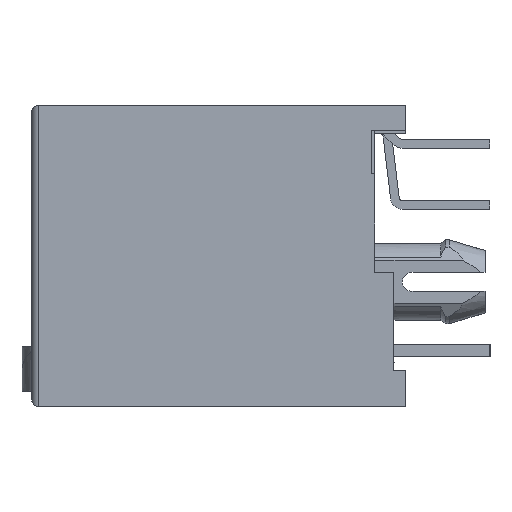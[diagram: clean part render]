
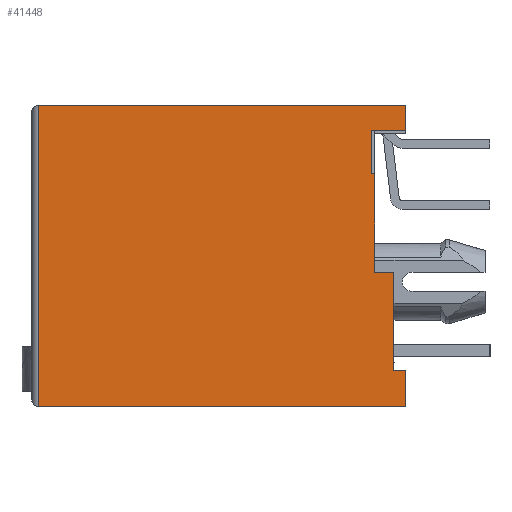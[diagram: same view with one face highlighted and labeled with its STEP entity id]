
A CAD part, left-side view. The second image highlights one B-rep face of the part: STEP entity #41448.
In plain terms, the highlighted planar face has unit normal (-1, 0, 0).
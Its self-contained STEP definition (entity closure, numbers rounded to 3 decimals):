
#1289 = CARTESIAN_POINT ( 'NONE',  ( -31.5, -7.8, -4.75 ) ) ;
#1361 = CARTESIAN_POINT ( 'NONE',  ( -31.5, -7.3, -2.017 ) ) ;
#2242 = ORIENTED_EDGE ( 'NONE', *, *, #23222, .F. ) ;
#2690 = CARTESIAN_POINT ( 'NONE',  ( -31.5, -7.8, 5.25 ) ) ;
#2831 = VERTEX_POINT ( 'NONE', #45628 ) ;
#3035 = VERTEX_POINT ( 'NONE', #38251 ) ;
#3059 = CARTESIAN_POINT ( 'NONE',  ( -31.5, -7.8, -4.75 ) ) ;
#3420 = CARTESIAN_POINT ( 'NONE',  ( -31.5, 2.4, -6.25 ) ) ;
#4001 = CARTESIAN_POINT ( 'NONE',  ( -31.5, -6.35, 3.45 ) ) ;
#9005 = VERTEX_POINT ( 'NONE', #67894 ) ;
#9206 = CARTESIAN_POINT ( 'NONE',  ( -31.5, -7.033, -0.65 ) ) ;
#9607 = EDGE_CURVE ( 'NONE', #9005, #52821, #56944, .T. ) ;
#10923 = B_SPLINE_CURVE_WITH_KNOTS ( 'NONE', 3,
 ( #65220, #17979, #29176, #18321 ),
 .UNSPECIFIED., .F., .F.,
 ( 4, 4 ),
 ( 0., 1. ),
 .UNSPECIFIED. ) ;
#11997 = ORIENTED_EDGE ( 'NONE', *, *, #55555, .F. ) ;
#12264 = ORIENTED_EDGE ( 'NONE', *, *, #9607, .F. ) ;
#12974 = EDGE_CURVE ( 'NONE', #28964, #3035, #21180, .T. ) ;
#13298 = ORIENTED_EDGE ( 'NONE', *, *, #45042, .F. ) ;
#13958 = CARTESIAN_POINT ( 'NONE',  ( -31.5, -7.8, -6.25 ) ) ;
#14138 = DIRECTION ( 'NONE',  ( 1., 0., 0. ) ) ;
#15414 = VERTEX_POINT ( 'NONE', #3059 ) ;
#15849 = EDGE_LOOP ( 'NONE', ( #11997, #13298, #56717, #12264, #29305, #52964, #27639, #54997, #2242, #47644, #48200, #30261 ) ) ;
#16614 = CARTESIAN_POINT ( 'NONE',  ( -31.5, -6.5, 3.45 ) ) ;
#16707 = B_SPLINE_CURVE_WITH_KNOTS ( 'NONE', 3,
 ( #13958, #35323, #3420, #68172 ),
 .UNSPECIFIED., .F., .F.,
 ( 4, 4 ),
 ( 0., 1. ),
 .UNSPECIFIED. ) ;
#17415 = CARTESIAN_POINT ( 'NONE',  ( -31.5, -7.633, -4.75 ) ) ;
#17540 = VERTEX_POINT ( 'NONE', #36992 ) ;
#17979 = CARTESIAN_POINT ( 'NONE',  ( -31.5, 7.5, 2.117 ) ) ;
#18321 = CARTESIAN_POINT ( 'NONE',  ( -31.5, 7.5, -6.25 ) ) ;
#18712 = FACE_OUTER_BOUND ( 'NONE', #15849, .T. ) ;
#19051 = EDGE_CURVE ( 'NONE', #2831, #23080, #10923, .T. ) ;
#19478 = EDGE_CURVE ( 'NONE', #65992, #2831, #42537, .T. ) ;
#19932 = CARTESIAN_POINT ( 'NONE',  ( -31.5, -6.45, 3.45 ) ) ;
#20110 = CARTESIAN_POINT ( 'NONE',  ( -31.5, -6.35, 5.25 ) ) ;
#20282 = CARTESIAN_POINT ( 'NONE',  ( -31.5, -6.4, 3.45 ) ) ;
#21180 = B_SPLINE_CURVE_WITH_KNOTS ( 'NONE', 3,
 ( #2690, #21926, #26493, #47478 ),
 .UNSPECIFIED., .F., .F.,
 ( 4, 4 ),
 ( 0., 1. ),
 .UNSPECIFIED. ) ;
#21926 = CARTESIAN_POINT ( 'NONE',  ( -31.5, -7.317, 5.25 ) ) ;
#22568 = CARTESIAN_POINT ( 'NONE',  ( -31.5, -7.8, 5.95 ) ) ;
#23080 = VERTEX_POINT ( 'NONE', #69085 ) ;
#23222 = EDGE_CURVE ( 'NONE', #65992, #28964, #29611, .T. ) ;
#23573 = EDGE_CURVE ( 'NONE', #52821, #56910, #57981, .T. ) ;
#23667 = CARTESIAN_POINT ( 'NONE',  ( -31.5, -7.8, -5.75 ) ) ;
#23926 = CARTESIAN_POINT ( 'NONE',  ( -31.5, -7.8, 5.25 ) ) ;
#25589 = CARTESIAN_POINT ( 'NONE',  ( -31.5, -6.35, 3.45 ) ) ;
#26236 = B_SPLINE_CURVE_WITH_KNOTS ( 'NONE', 3,
 ( #20110, #56537, #62806, #4001 ),
 .UNSPECIFIED., .F., .F.,
 ( 4, 4 ),
 ( 0., 1. ),
 .UNSPECIFIED. ) ;
#26493 = CARTESIAN_POINT ( 'NONE',  ( -31.5, -6.833, 5.25 ) ) ;
#26725 = EDGE_CURVE ( 'NONE', #44472, #47911, #36726, .T. ) ;
#27639 = ORIENTED_EDGE ( 'NONE', *, *, #55695, .F. ) ;
#28177 = CARTESIAN_POINT ( 'NONE',  ( -31.5, -7.8, 5.25 ) ) ;
#28919 = CARTESIAN_POINT ( 'NONE',  ( -31.5, -7.8, -5.25 ) ) ;
#28964 = VERTEX_POINT ( 'NONE', #23926 ) ;
#29176 = CARTESIAN_POINT ( 'NONE',  ( -31.5, 7.5, -2.067 ) ) ;
#29305 = ORIENTED_EDGE ( 'NONE', *, *, #69170, .F. ) ;
#29611 = B_SPLINE_CURVE_WITH_KNOTS ( 'NONE', 3,
 ( #58958, #22568, #43231, #28177 ),
 .UNSPECIFIED., .F., .F.,
 ( 4, 4 ),
 ( 0., 1. ),
 .UNSPECIFIED. ) ;
#30261 = ORIENTED_EDGE ( 'NONE', *, *, #34553, .F. ) ;
#31166 = AXIS2_PLACEMENT_3D ( 'NONE', #40754, #14138, #35502 ) ;
#33802 = CARTESIAN_POINT ( 'NONE',  ( -31.5, -6.5, 0.717 ) ) ;
#34553 = EDGE_CURVE ( 'NONE', #17540, #23080, #16707, .T. ) ;
#35323 = CARTESIAN_POINT ( 'NONE',  ( -31.5, -2.7, -6.25 ) ) ;
#35502 = DIRECTION ( 'NONE',  ( 0., 0., 1. ) ) ;
#35832 = CARTESIAN_POINT ( 'NONE',  ( -31.5, -6.5, -0.65 ) ) ;
#36726 = B_SPLINE_CURVE_WITH_KNOTS ( 'NONE', 3,
 ( #68205, #20282, #19932, #68551 ),
 .UNSPECIFIED., .F., .F.,
 ( 4, 4 ),
 ( 0., 1. ),
 .UNSPECIFIED. ) ;
#36861 = CARTESIAN_POINT ( 'NONE',  ( -31.5, -7.3, -0.65 ) ) ;
#36992 = CARTESIAN_POINT ( 'NONE',  ( -31.5, -7.8, -6.25 ) ) ;
#38251 = CARTESIAN_POINT ( 'NONE',  ( -31.5, -6.35, 5.25 ) ) ;
#38496 = CARTESIAN_POINT ( 'NONE',  ( -31.5, -7.3, -4.75 ) ) ;
#38780 = CARTESIAN_POINT ( 'NONE',  ( -31.5, -7.467, -4.75 ) ) ;
#39735 = CARTESIAN_POINT ( 'NONE',  ( -31.5, -6.5, -0.65 ) ) ;
#40754 = CARTESIAN_POINT ( 'NONE',  ( -31.5, 7.806, -6.501 ) ) ;
#41448 = ADVANCED_FACE ( 'NONE', ( #18712 ), #61732, .F. ) ;
#42120 = CARTESIAN_POINT ( 'NONE',  ( -31.5, 7.5, 6.3 ) ) ;
#42537 = B_SPLINE_CURVE_WITH_KNOTS ( 'NONE', 3,
 ( #46295, #63077, #62734, #42120 ),
 .UNSPECIFIED., .F., .F.,
 ( 4, 4 ),
 ( 0., 1. ),
 .UNSPECIFIED. ) ;
#43231 = CARTESIAN_POINT ( 'NONE',  ( -31.5, -7.8, 5.6 ) ) ;
#44472 = VERTEX_POINT ( 'NONE', #25589 ) ;
#45042 = EDGE_CURVE ( 'NONE', #56910, #15414, #51610, .T. ) ;
#45628 = CARTESIAN_POINT ( 'NONE',  ( -31.5, 7.5, 6.3 ) ) ;
#45699 = CARTESIAN_POINT ( 'NONE',  ( -31.5, -7.8, -4.75 ) ) ;
#46295 = CARTESIAN_POINT ( 'NONE',  ( -31.5, -7.8, 6.3 ) ) ;
#47478 = CARTESIAN_POINT ( 'NONE',  ( -31.5, -6.35, 5.25 ) ) ;
#47644 = ORIENTED_EDGE ( 'NONE', *, *, #19478, .T. ) ;
#47911 = VERTEX_POINT ( 'NONE', #16614 ) ;
#48200 = ORIENTED_EDGE ( 'NONE', *, *, #19051, .T. ) ;
#49001 = CARTESIAN_POINT ( 'NONE',  ( -31.5, -7.3, -0.65 ) ) ;
#49268 = CARTESIAN_POINT ( 'NONE',  ( -31.5, -7.3, -4.75 ) ) ;
#50349 = CARTESIAN_POINT ( 'NONE',  ( -31.5, -7.3, -3.383 ) ) ;
#50574 = CARTESIAN_POINT ( 'NONE',  ( -31.5, -7.8, 6.3 ) ) ;
#50857 = CARTESIAN_POINT ( 'NONE',  ( -31.5, -7.3, -4.75 ) ) ;
#51610 = B_SPLINE_CURVE_WITH_KNOTS ( 'NONE', 3,
 ( #49268, #38780, #17415, #1289 ),
 .UNSPECIFIED., .F., .F.,
 ( 4, 4 ),
 ( 0., 1. ),
 .UNSPECIFIED. ) ;
#52691 = B_SPLINE_CURVE_WITH_KNOTS ( 'NONE', 3,
 ( #54775, #60372, #33802, #39735 ),
 .UNSPECIFIED., .F., .F.,
 ( 4, 4 ),
 ( 0., 1. ),
 .UNSPECIFIED. ) ;
#52821 = VERTEX_POINT ( 'NONE', #68323 ) ;
#52964 = ORIENTED_EDGE ( 'NONE', *, *, #26725, .F. ) ;
#54613 = B_SPLINE_CURVE_WITH_KNOTS ( 'NONE', 3,
 ( #45699, #28919, #23667, #65649 ),
 .UNSPECIFIED., .F., .F.,
 ( 4, 4 ),
 ( 0., 1. ),
 .UNSPECIFIED. ) ;
#54775 = CARTESIAN_POINT ( 'NONE',  ( -31.5, -6.5, 3.45 ) ) ;
#54997 = ORIENTED_EDGE ( 'NONE', *, *, #12974, .F. ) ;
#55555 = EDGE_CURVE ( 'NONE', #15414, #17540, #54613, .T. ) ;
#55695 = EDGE_CURVE ( 'NONE', #3035, #44472, #26236, .T. ) ;
#56537 = CARTESIAN_POINT ( 'NONE',  ( -31.5, -6.35, 4.65 ) ) ;
#56717 = ORIENTED_EDGE ( 'NONE', *, *, #23573, .F. ) ;
#56910 = VERTEX_POINT ( 'NONE', #50857 ) ;
#56944 = B_SPLINE_CURVE_WITH_KNOTS ( 'NONE', 3,
 ( #35832, #57162, #9206, #36861 ),
 .UNSPECIFIED., .F., .F.,
 ( 4, 4 ),
 ( 0., 1. ),
 .UNSPECIFIED. ) ;
#57162 = CARTESIAN_POINT ( 'NONE',  ( -31.5, -6.767, -0.65 ) ) ;
#57981 = B_SPLINE_CURVE_WITH_KNOTS ( 'NONE', 3,
 ( #49001, #1361, #50349, #38496 ),
 .UNSPECIFIED., .F., .F.,
 ( 4, 4 ),
 ( 0., 1. ),
 .UNSPECIFIED. ) ;
#58958 = CARTESIAN_POINT ( 'NONE',  ( -31.5, -7.8, 6.3 ) ) ;
#60372 = CARTESIAN_POINT ( 'NONE',  ( -31.5, -6.5, 2.083 ) ) ;
#61732 = PLANE ( 'NONE',  #31166 ) ;
#62734 = CARTESIAN_POINT ( 'NONE',  ( -31.5, 2.4, 6.3 ) ) ;
#62806 = CARTESIAN_POINT ( 'NONE',  ( -31.5, -6.35, 4.05 ) ) ;
#63077 = CARTESIAN_POINT ( 'NONE',  ( -31.5, -2.7, 6.3 ) ) ;
#65220 = CARTESIAN_POINT ( 'NONE',  ( -31.5, 7.5, 6.3 ) ) ;
#65649 = CARTESIAN_POINT ( 'NONE',  ( -31.5, -7.8, -6.25 ) ) ;
#65992 = VERTEX_POINT ( 'NONE', #50574 ) ;
#67894 = CARTESIAN_POINT ( 'NONE',  ( -31.5, -6.5, -0.65 ) ) ;
#68172 = CARTESIAN_POINT ( 'NONE',  ( -31.5, 7.5, -6.25 ) ) ;
#68205 = CARTESIAN_POINT ( 'NONE',  ( -31.5, -6.35, 3.45 ) ) ;
#68323 = CARTESIAN_POINT ( 'NONE',  ( -31.5, -7.3, -0.65 ) ) ;
#68551 = CARTESIAN_POINT ( 'NONE',  ( -31.5, -6.5, 3.45 ) ) ;
#69085 = CARTESIAN_POINT ( 'NONE',  ( -31.5, 7.5, -6.25 ) ) ;
#69170 = EDGE_CURVE ( 'NONE', #47911, #9005, #52691, .T. ) ;
